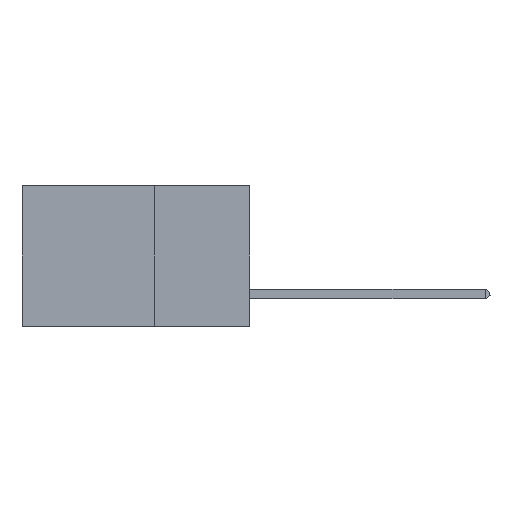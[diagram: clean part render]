
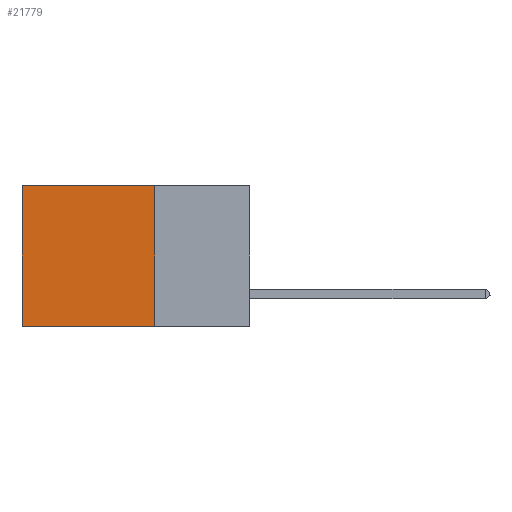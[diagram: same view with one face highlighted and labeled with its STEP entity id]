
A CAD part, left-side view. The second image highlights one B-rep face of the part: STEP entity #21779.
In plain terms, the highlighted planar face has unit normal (-1, 0, 0).
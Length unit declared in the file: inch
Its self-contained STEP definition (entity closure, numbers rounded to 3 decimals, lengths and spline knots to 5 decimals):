
#644 = LINE ( 'NONE', #32929, #24157 ) ;
#1842 = VERTEX_POINT ( 'NONE', #9098 ) ;
#2194 = CARTESIAN_POINT ( 'NONE',  ( 0.2875, 0.6, -0.37 ) ) ;
#2270 = PLANE ( 'NONE',  #38091 ) ;
#4595 = LINE ( 'NONE', #7314, #24329 ) ;
#4987 = LINE ( 'NONE', #37145, #23210 ) ;
#5599 = DIRECTION ( 'NONE',  ( 0., 1., 0. ) ) ;
#5759 = CARTESIAN_POINT ( 'NONE',  ( 0.2875, 0.25, 0. ) ) ;
#6151 = DIRECTION ( 'NONE',  ( 0., 0., -1. ) ) ;
#7314 = CARTESIAN_POINT ( 'NONE',  ( 0.2875, 0.25, -0.37 ) ) ;
#9098 = CARTESIAN_POINT ( 'NONE',  ( 0.2875, 0.25, -0.37 ) ) ;
#9809 = FACE_OUTER_BOUND ( 'NONE', #15002, .T. ) ;
#11507 = DIRECTION ( 'NONE',  ( 1., 0., 0. ) ) ;
#12513 = CARTESIAN_POINT ( 'NONE',  ( 0.2875, 0.6, 0. ) ) ;
#13458 = DIRECTION ( 'NONE',  ( 0., 1., 0. ) ) ;
#15002 = EDGE_LOOP ( 'NONE', ( #21294, #25835, #19288, #20589 ) ) ;
#18622 = DIRECTION ( 'NONE',  ( 0., 0., -1. ) ) ;
#19288 = ORIENTED_EDGE ( 'NONE', *, *, #27214, .F. ) ;
#20589 = ORIENTED_EDGE ( 'NONE', *, *, #35937, .T. ) ;
#21294 = ORIENTED_EDGE ( 'NONE', *, *, #21553, .T. ) ;
#21553 = EDGE_CURVE ( 'NONE', #36279, #34172, #4987, .T. ) ;
#21779 = ADVANCED_FACE ( 'NONE', ( #9809 ), #2270, .F. ) ;
#23210 = VECTOR ( 'NONE', #18622, 39.37008 ) ;
#24157 = VECTOR ( 'NONE', #5599, 39.37008 ) ;
#24263 = CARTESIAN_POINT ( 'NONE',  ( 0.2875, 0.25, 0. ) ) ;
#24329 = VECTOR ( 'NONE', #13458, 39.37008 ) ;
#25312 = VERTEX_POINT ( 'NONE', #5759 ) ;
#25492 = EDGE_CURVE ( 'NONE', #1842, #34172, #4595, .T. ) ;
#25835 = ORIENTED_EDGE ( 'NONE', *, *, #25492, .F. ) ;
#27214 = EDGE_CURVE ( 'NONE', #25312, #1842, #27619, .T. ) ;
#27619 = LINE ( 'NONE', #24263, #29960 ) ;
#29918 = CARTESIAN_POINT ( 'NONE',  ( 0.2875, 0.25, 0. ) ) ;
#29960 = VECTOR ( 'NONE', #6151, 39.37008 ) ;
#32929 = CARTESIAN_POINT ( 'NONE',  ( 0.2875, 0.25, 0. ) ) ;
#33253 = DIRECTION ( 'NONE',  ( 0., 0., -1. ) ) ;
#34172 = VERTEX_POINT ( 'NONE', #2194 ) ;
#35937 = EDGE_CURVE ( 'NONE', #25312, #36279, #644, .T. ) ;
#36279 = VERTEX_POINT ( 'NONE', #12513 ) ;
#37145 = CARTESIAN_POINT ( 'NONE',  ( 0.2875, 0.6, 0. ) ) ;
#38091 = AXIS2_PLACEMENT_3D ( 'NONE', #29918, #11507, #33253 ) ;
